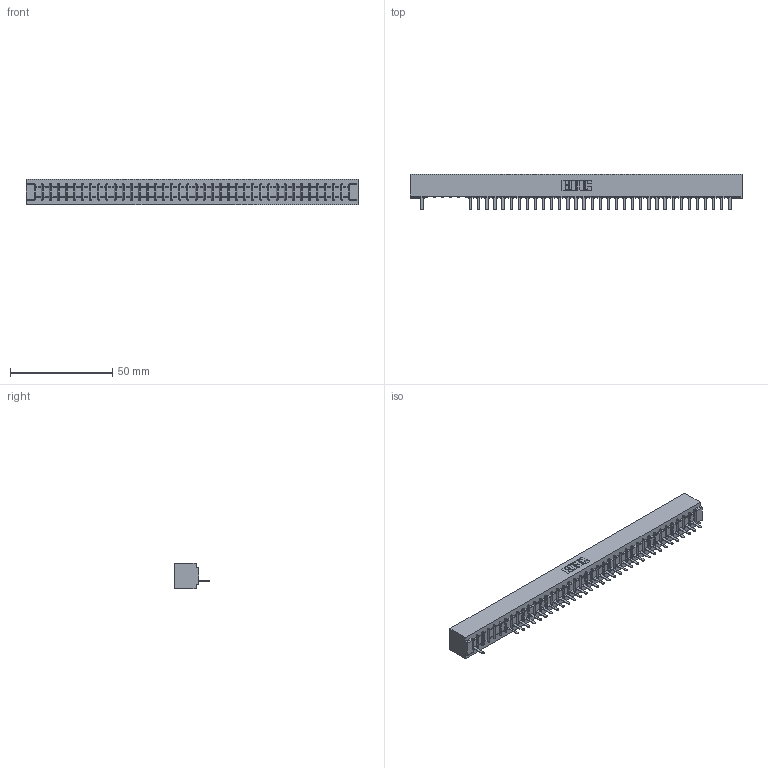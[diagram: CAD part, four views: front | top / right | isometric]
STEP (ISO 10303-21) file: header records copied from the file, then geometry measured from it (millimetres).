
FILE_DESCRIPTION (( 'STEP AP203' ), '1' );
FILE_NAME ('357-039-521-101.STEP', '2018-08-10T11:44:27', ( '' ), ( '' ), 'SwSTEP 2.0', 'SolidWorks 2016', '' );
FILE_SCHEMA (( 'CONFIG_CONTROL_DESIGN' ));
Length unit declared in the file: inch
Products named in the file (3): 307 Part_No Mounting Lugs; 307-290-002_521; 357-039-521-101
Assembly tree (35 placements, depth 2):
  357-039-521-101
    307 Part_No Mounting Lugs
    307-290-002_521  x34
Bounding box: 162.41 x 17.42 x 12.7 mm (x, y, z)
Volume: 17772.4 mm3; surface area: 21709.1 mm2
Topology: 35 solids, 35 shells, 2766 faces, 8507 edges, 5562 vertices
Faces by surface type: plane 1656, cylinder 1030, sphere 80
Entity records: 34084 total; most frequent: CARTESIAN_POINT 5771, ORIENTED_EDGE 5766, DIRECTION 5601, EDGE_CURVE 2883, LINE 2209, VECTOR 2209, VERTEX_POINT 1866, AXIS2_PLACEMENT_3D 1696
